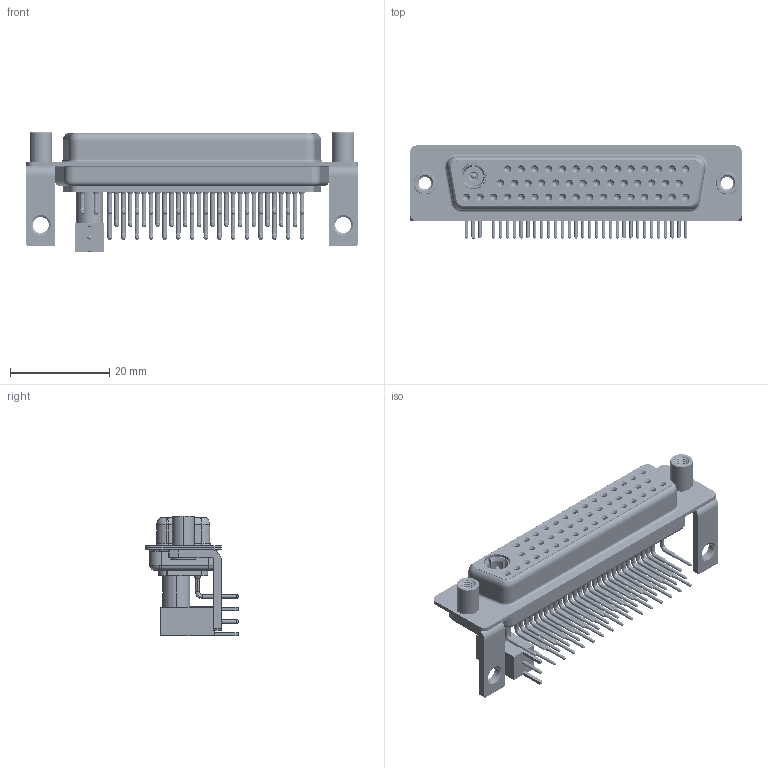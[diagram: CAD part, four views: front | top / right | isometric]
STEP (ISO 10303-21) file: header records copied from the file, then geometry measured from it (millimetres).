
FILE_DESCRIPTION (( 'STEP AP203' ), '1' );
FILE_NAME ('630-47W1640-5N6.STEP', '2022-06-10T13:15:40', ( '' ), ( '' ), 'SwSTEP 2.0', 'SolidWorks 2020', '' );
FILE_SCHEMA (( 'CONFIG_CONTROL_DESIGN' ));
Length unit declared in the file: millimetre
Products named in the file (16): 630Combo Contact Row 3; Pin_RA 50; 630-47W1640-5N6; Locking Collar; 630Combo Threaded Standoff_D; RA Back Shell_50; 630Combo Shell Front_50 Contacts; 630Combo Contact Row 1_50 Contacts; 630Combo Stabilizer Bracket_50 Contacts; Insulator Pin_Straight PC Tail; 630Combo Shell Rear_50 Contacts; Co-Ax Plug Assy_RA 50; 630Combo Housing_47W1; Co-Ax Plug_RA 50; 630Combo Contact Row 2_50 Contacts; Insulator RA Pin
Assembly tree (60 placements, depth 3):
  630-47W1640-5N6
    630Combo Housing_47W1
    630Combo Shell Front_50 Contacts
    630Combo Shell Rear_50 Contacts
    630Combo Stabilizer Bracket_50 Contacts  x2
    630Combo Threaded Standoff_D  x2
    Co-Ax Plug Assy_RA 50
      Co-Ax Plug_RA 50
      Insulator Pin_Straight PC Tail
      Pin_RA 50
      Locking Collar
      RA Back Shell_50
      Insulator RA Pin
    630Combo Contact Row 1_50 Contacts  x15
    630Combo Contact Row 2_50 Contacts  x14
    630Combo Contact Row 3  x17
Bounding box: 67 x 18.8 x 24.16 mm (x, y, z)
Volume: 7976.2 mm3; surface area: 17837.8 mm2
Topology: 59 solids, 59 shells, 2970 faces, 7538 edges, 4748 vertices
Faces by surface type: cylinder 1324, plane 843, cone 545, bspline 191, torus 63, sphere 4
Entity records: 39465 total; most frequent: CARTESIAN_POINT 8666, DIRECTION 6414, ORIENTED_EDGE 5394, EDGE_CURVE 2697, AXIS2_PLACEMENT_3D 2671, VERTEX_POINT 1724, CIRCLE 1455, EDGE_LOOP 1453
